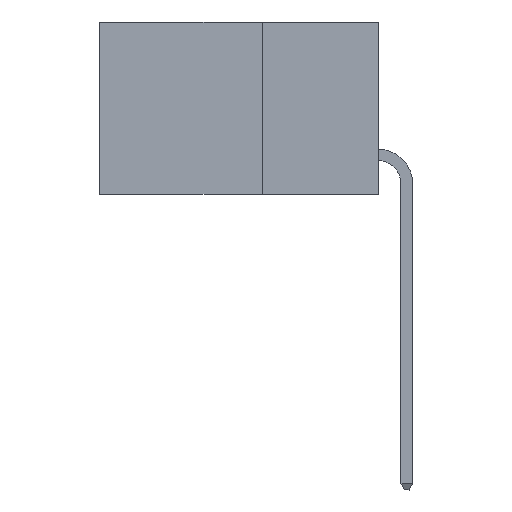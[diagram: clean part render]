
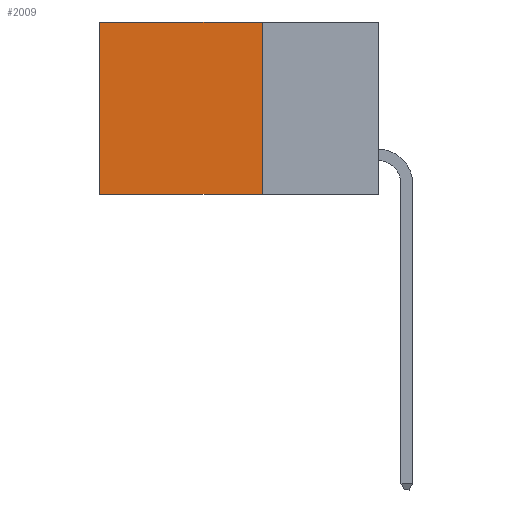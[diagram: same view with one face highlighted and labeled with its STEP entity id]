
A CAD part, left-side view. The second image highlights one B-rep face of the part: STEP entity #2009.
In plain terms, the highlighted planar face has unit normal (-1, 0, 0).
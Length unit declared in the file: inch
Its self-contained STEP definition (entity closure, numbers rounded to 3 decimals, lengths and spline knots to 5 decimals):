
#1088 = AXIS2_PLACEMENT_3D ( 'NONE', #8935, #3669, #9301 ) ;
#1180 = VERTEX_POINT ( 'NONE', #16745 ) ;
#1998 = CARTESIAN_POINT ( 'NONE',  ( 0.2615, 0.25, -0.37 ) ) ;
#2009 = ADVANCED_FACE ( 'NONE', ( #22635 ), #3317, .F. ) ;
#2103 = ORIENTED_EDGE ( 'NONE', *, *, #23825, .F. ) ;
#2142 = EDGE_CURVE ( 'NONE', #4064, #8061, #6492, .T. ) ;
#2464 = VECTOR ( 'NONE', #20986, 39.37008 ) ;
#2647 = ORIENTED_EDGE ( 'NONE', *, *, #2142, .T. ) ;
#3317 = PLANE ( 'NONE',  #1088 ) ;
#3669 = DIRECTION ( 'NONE',  ( 1., 0., 0. ) ) ;
#4064 = VERTEX_POINT ( 'NONE', #17895 ) ;
#4511 = VERTEX_POINT ( 'NONE', #12300 ) ;
#4930 = EDGE_CURVE ( 'NONE', #4064, #4511, #24721, .T. ) ;
#6170 = CARTESIAN_POINT ( 'NONE',  ( 0.2615, 0.6, -0.37 ) ) ;
#6492 = LINE ( 'NONE', #10234, #15071 ) ;
#8035 = CARTESIAN_POINT ( 'NONE',  ( 0.2615, 0.25, -0.37 ) ) ;
#8061 = VERTEX_POINT ( 'NONE', #14906 ) ;
#8768 = EDGE_LOOP ( 'NONE', ( #21216, #2103, #21725, #2647 ) ) ;
#8935 = CARTESIAN_POINT ( 'NONE',  ( 0.2615, 0.25, -0.37 ) ) ;
#9301 = DIRECTION ( 'NONE',  ( 0., 0., -1. ) ) ;
#9388 = DIRECTION ( 'NONE',  ( 0., 0., -1. ) ) ;
#10234 = CARTESIAN_POINT ( 'NONE',  ( 0.2615, 0.25, 0. ) ) ;
#11400 = DIRECTION ( 'NONE',  ( 0., 1., 0. ) ) ;
#12300 = CARTESIAN_POINT ( 'NONE',  ( 0.2615, 0.25, -0.37 ) ) ;
#14064 = DIRECTION ( 'NONE',  ( 0., 0., -1. ) ) ;
#14906 = CARTESIAN_POINT ( 'NONE',  ( 0.2615, 0.6, 0. ) ) ;
#15071 = VECTOR ( 'NONE', #11400, 39.37008 ) ;
#16745 = CARTESIAN_POINT ( 'NONE',  ( 0.2615, 0.6, -0.37 ) ) ;
#17895 = CARTESIAN_POINT ( 'NONE',  ( 0.2615, 0.25, 0. ) ) ;
#19206 = VECTOR ( 'NONE', #9388, 39.37008 ) ;
#20009 = VECTOR ( 'NONE', #14064, 39.37008 ) ;
#20986 = DIRECTION ( 'NONE',  ( 0., 1., 0. ) ) ;
#21216 = ORIENTED_EDGE ( 'NONE', *, *, #22074, .T. ) ;
#21725 = ORIENTED_EDGE ( 'NONE', *, *, #4930, .F. ) ;
#22074 = EDGE_CURVE ( 'NONE', #8061, #1180, #23643, .T. ) ;
#22635 = FACE_OUTER_BOUND ( 'NONE', #8768, .T. ) ;
#22760 = LINE ( 'NONE', #8035, #2464 ) ;
#23643 = LINE ( 'NONE', #6170, #20009 ) ;
#23825 = EDGE_CURVE ( 'NONE', #4511, #1180, #22760, .T. ) ;
#24721 = LINE ( 'NONE', #1998, #19206 ) ;
